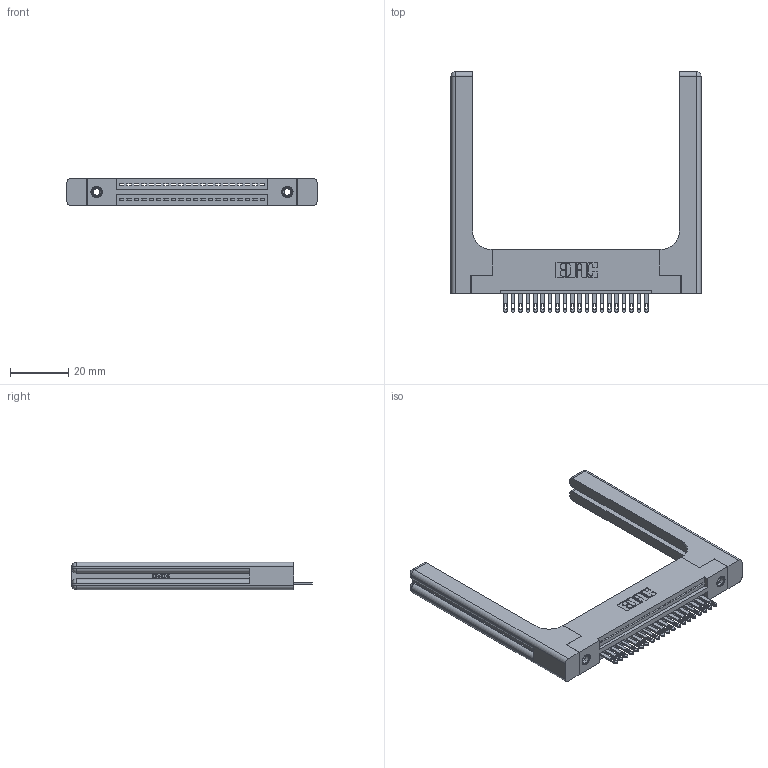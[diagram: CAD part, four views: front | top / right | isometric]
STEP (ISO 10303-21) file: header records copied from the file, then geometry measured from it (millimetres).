
FILE_DESCRIPTION (( 'STEP AP203' ), '1' );
FILE_NAME ('345-020-500-158.STEP', '2019-10-04T19:54:12', ( '' ), ( '' ), 'SwSTEP 2.0', 'SolidWorks 2016', '' );
FILE_SCHEMA (( 'CONFIG_CONTROL_DESIGN' ));
Length unit declared in the file: inch
Products named in the file (5): 345-220-058_345-220-058; 345-292-001_345-293-100; 345 Part_Flush Mounting Lugs - 0.156 Dia-TH; 345-020-500-158; 345-250-001_345-250-001-102
Assembly tree (25 placements, depth 2):
  345-020-500-158
    345 Part_Flush Mounting Lugs - 0.156 Dia-TH
    345-292-001_345-293-100  x20
    345-250-001_345-250-001-102  x2
    345-220-058_345-220-058  x2
Bounding box: 85.83 x 82.47 x 9.4 mm (x, y, z)
Volume: 16489 mm3; surface area: 15661.6 mm2
Topology: 25 solids, 25 shells, 1462 faces, 4367 edges, 2890 vertices
Faces by surface type: plane 908, cylinder 494, bspline 36, cone 12, sphere 8, torus 4
Entity records: 23126 total; most frequent: CARTESIAN_POINT 4977, ORIENTED_EDGE 3728, DIRECTION 3328, EDGE_CURVE 1864, VECTOR 1556, LINE 1556, VERTEX_POINT 1234, AXIS2_PLACEMENT_3D 886
